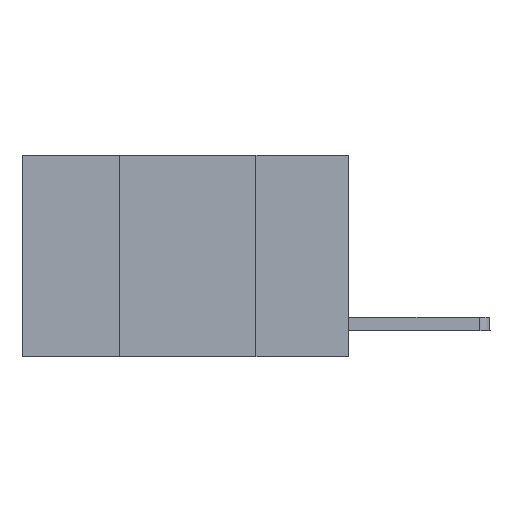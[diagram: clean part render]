
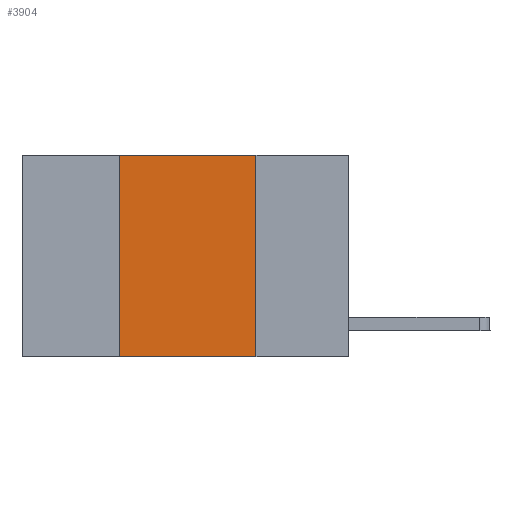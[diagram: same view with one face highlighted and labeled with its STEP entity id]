
A CAD part, left-side view. The second image highlights one B-rep face of the part: STEP entity #3904.
In plain terms, the highlighted planar face has unit normal (-1, 0, 0).
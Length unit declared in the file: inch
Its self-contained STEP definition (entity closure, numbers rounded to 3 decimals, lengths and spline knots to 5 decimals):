
#200 = ORIENTED_EDGE ( 'NONE', *, *, #9763, .F. ) ;
#232 = DIRECTION ( 'NONE',  ( 0., -1., 0. ) ) ;
#402 = PLANE ( 'NONE',  #3827 ) ;
#484 = DIRECTION ( 'NONE',  ( 1., 0., 0. ) ) ;
#850 = VERTEX_POINT ( 'NONE', #3116 ) ;
#900 = CARTESIAN_POINT ( 'NONE',  ( 0., 0.42, -0.37 ) ) ;
#1025 = LINE ( 'NONE', #4002, #7328 ) ;
#1573 = CARTESIAN_POINT ( 'NONE',  ( 0., 0.17, 0. ) ) ;
#1795 = FACE_OUTER_BOUND ( 'NONE', #4711, .T. ) ;
#2363 = VECTOR ( 'NONE', #8642, 39.37008 ) ;
#2710 = ORIENTED_EDGE ( 'NONE', *, *, #6153, .F. ) ;
#2769 = ORIENTED_EDGE ( 'NONE', *, *, #9453, .T. ) ;
#2871 = CARTESIAN_POINT ( 'NONE',  ( 0., 0.17, 0. ) ) ;
#2937 = CARTESIAN_POINT ( 'NONE',  ( 0., 0.6, -0.37 ) ) ;
#2987 = LINE ( 'NONE', #2937, #6637 ) ;
#3116 = CARTESIAN_POINT ( 'NONE',  ( 0., 0.42, 0. ) ) ;
#3827 = AXIS2_PLACEMENT_3D ( 'NONE', #6566, #484, #4986 ) ;
#3904 = ADVANCED_FACE ( 'NONE', ( #1795 ), #402, .F. ) ;
#4002 = CARTESIAN_POINT ( 'NONE',  ( 0., 0.6, 0. ) ) ;
#4281 = DIRECTION ( 'NONE',  ( 0., 0., -1. ) ) ;
#4711 = EDGE_LOOP ( 'NONE', ( #2710, #9302, #200, #2769 ) ) ;
#4852 = EDGE_CURVE ( 'NONE', #850, #7266, #1025, .T. ) ;
#4986 = DIRECTION ( 'NONE',  ( 0., 0., -1. ) ) ;
#5156 = LINE ( 'NONE', #2871, #5749 ) ;
#5255 = CARTESIAN_POINT ( 'NONE',  ( 0., 0.17, -0.37 ) ) ;
#5749 = VECTOR ( 'NONE', #4281, 39.37008 ) ;
#6153 = EDGE_CURVE ( 'NONE', #7266, #8658, #5156, .T. ) ;
#6458 = CARTESIAN_POINT ( 'NONE',  ( 0., 0.42, 0. ) ) ;
#6500 = LINE ( 'NONE', #6458, #2363 ) ;
#6566 = CARTESIAN_POINT ( 'NONE',  ( 0., 0.6, 0. ) ) ;
#6637 = VECTOR ( 'NONE', #9647, 39.37008 ) ;
#6741 = VERTEX_POINT ( 'NONE', #900 ) ;
#7266 = VERTEX_POINT ( 'NONE', #1573 ) ;
#7328 = VECTOR ( 'NONE', #232, 39.37008 ) ;
#8642 = DIRECTION ( 'NONE',  ( 0., 0., 1. ) ) ;
#8658 = VERTEX_POINT ( 'NONE', #5255 ) ;
#9302 = ORIENTED_EDGE ( 'NONE', *, *, #4852, .F. ) ;
#9453 = EDGE_CURVE ( 'NONE', #6741, #8658, #2987, .T. ) ;
#9647 = DIRECTION ( 'NONE',  ( 0., -1., 0. ) ) ;
#9763 = EDGE_CURVE ( 'NONE', #6741, #850, #6500, .T. ) ;
